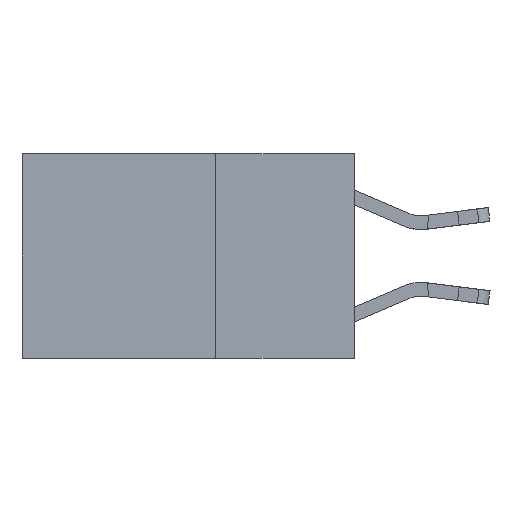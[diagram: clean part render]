
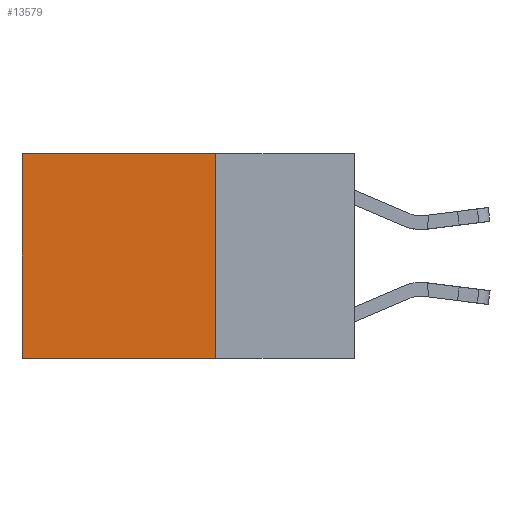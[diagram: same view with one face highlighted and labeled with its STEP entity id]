
A CAD part, left-side view. The second image highlights one B-rep face of the part: STEP entity #13579.
In plain terms, the highlighted planar face has unit normal (-1, 0, 0).
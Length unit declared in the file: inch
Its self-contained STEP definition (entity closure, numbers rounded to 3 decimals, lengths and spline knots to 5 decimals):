
#311 = VECTOR ( 'NONE', #8635, 39.37008 ) ;
#1516 = EDGE_CURVE ( 'NONE', #17512, #11166, #2086, .T. ) ;
#1893 = DIRECTION ( 'NONE',  ( 0., 0., -1. ) ) ;
#2086 = LINE ( 'NONE', #8198, #16772 ) ;
#2250 = VECTOR ( 'NONE', #12461, 39.37008 ) ;
#2530 = DIRECTION ( 'NONE',  ( 1., 0., 0. ) ) ;
#2574 = EDGE_CURVE ( 'NONE', #8792, #11166, #15693, .T. ) ;
#4749 = LINE ( 'NONE', #16812, #311 ) ;
#4845 = FACE_OUTER_BOUND ( 'NONE', #6069, .T. ) ;
#6069 = EDGE_LOOP ( 'NONE', ( #16211, #8172, #11650, #13571 ) ) ;
#7381 = CARTESIAN_POINT ( 'NONE',  ( 0.2625, 0.25, 0. ) ) ;
#7743 = CARTESIAN_POINT ( 'NONE',  ( 0.2625, 0.6, 0. ) ) ;
#8172 = ORIENTED_EDGE ( 'NONE', *, *, #1516, .F. ) ;
#8198 = CARTESIAN_POINT ( 'NONE',  ( 0.2625, 0.25, -0.37 ) ) ;
#8635 = DIRECTION ( 'NONE',  ( 0., 0., -1. ) ) ;
#8792 = VERTEX_POINT ( 'NONE', #7743 ) ;
#9296 = DIRECTION ( 'NONE',  ( 0., 0., -1. ) ) ;
#11099 = CARTESIAN_POINT ( 'NONE',  ( 0.2625, 0.25, 0. ) ) ;
#11166 = VERTEX_POINT ( 'NONE', #15909 ) ;
#11417 = DIRECTION ( 'NONE',  ( 0., 1., 0. ) ) ;
#11650 = ORIENTED_EDGE ( 'NONE', *, *, #20367, .F. ) ;
#12323 = AXIS2_PLACEMENT_3D ( 'NONE', #11099, #2530, #9296 ) ;
#12461 = DIRECTION ( 'NONE',  ( 0., 1., 0. ) ) ;
#12564 = EDGE_CURVE ( 'NONE', #18604, #8792, #15409, .T. ) ;
#13571 = ORIENTED_EDGE ( 'NONE', *, *, #12564, .T. ) ;
#13579 = ADVANCED_FACE ( 'NONE', ( #4845 ), #17770, .F. ) ;
#13925 = CARTESIAN_POINT ( 'NONE',  ( 0.2625, 0.6, 0. ) ) ;
#14716 = CARTESIAN_POINT ( 'NONE',  ( 0.2625, 0.25, 0. ) ) ;
#15409 = LINE ( 'NONE', #7381, #2250 ) ;
#15693 = LINE ( 'NONE', #13925, #17781 ) ;
#15909 = CARTESIAN_POINT ( 'NONE',  ( 0.2625, 0.6, -0.37 ) ) ;
#16211 = ORIENTED_EDGE ( 'NONE', *, *, #2574, .T. ) ;
#16772 = VECTOR ( 'NONE', #11417, 39.37008 ) ;
#16812 = CARTESIAN_POINT ( 'NONE',  ( 0.2625, 0.25, 0. ) ) ;
#17512 = VERTEX_POINT ( 'NONE', #18599 ) ;
#17770 = PLANE ( 'NONE',  #12323 ) ;
#17781 = VECTOR ( 'NONE', #1893, 39.37008 ) ;
#18599 = CARTESIAN_POINT ( 'NONE',  ( 0.2625, 0.25, -0.37 ) ) ;
#18604 = VERTEX_POINT ( 'NONE', #14716 ) ;
#20367 = EDGE_CURVE ( 'NONE', #18604, #17512, #4749, .T. ) ;
